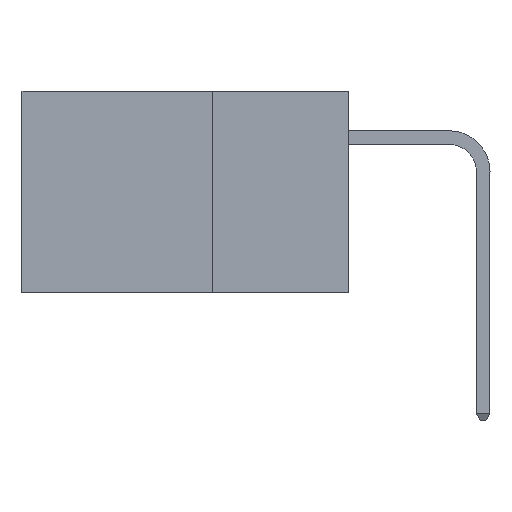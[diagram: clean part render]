
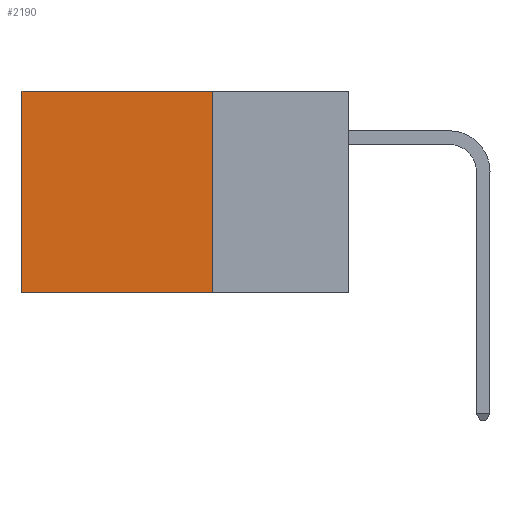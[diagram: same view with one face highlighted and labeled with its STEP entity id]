
A CAD part, left-side view. The second image highlights one B-rep face of the part: STEP entity #2190.
In plain terms, the highlighted planar face has unit normal (-1, 0, 0).
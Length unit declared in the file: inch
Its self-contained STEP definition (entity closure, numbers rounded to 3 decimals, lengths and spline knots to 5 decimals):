
#716 = CARTESIAN_POINT ( 'NONE',  ( 0.2875, 0.25, 0. ) ) ;
#831 = ORIENTED_EDGE ( 'NONE', *, *, #10721, .F. ) ;
#846 = DIRECTION ( 'NONE',  ( 0., 0., -1. ) ) ;
#870 = PLANE ( 'NONE',  #3968 ) ;
#1018 = DIRECTION ( 'NONE',  ( 1., 0., 0. ) ) ;
#1345 = ORIENTED_EDGE ( 'NONE', *, *, #7402, .T. ) ;
#1451 = EDGE_CURVE ( 'NONE', #5109, #9148, #7935, .T. ) ;
#1776 = CARTESIAN_POINT ( 'NONE',  ( 0.2875, 0.25, 0. ) ) ;
#1866 = CARTESIAN_POINT ( 'NONE',  ( 0.2875, 0.25, -0.37 ) ) ;
#1911 = DIRECTION ( 'NONE',  ( 0., 1., 0. ) ) ;
#2157 = CARTESIAN_POINT ( 'NONE',  ( 0.2875, 0.25, -0.37 ) ) ;
#2190 = ADVANCED_FACE ( 'NONE', ( #4365 ), #870, .F. ) ;
#2491 = CARTESIAN_POINT ( 'NONE',  ( 0.2875, 0.25, 0. ) ) ;
#3054 = DIRECTION ( 'NONE',  ( 0., 0., -1. ) ) ;
#3968 = AXIS2_PLACEMENT_3D ( 'NONE', #716, #1018, #846 ) ;
#4000 = DIRECTION ( 'NONE',  ( 0., 1., 0. ) ) ;
#4074 = ORIENTED_EDGE ( 'NONE', *, *, #1451, .F. ) ;
#4365 = FACE_OUTER_BOUND ( 'NONE', #11638, .T. ) ;
#4418 = VERTEX_POINT ( 'NONE', #7080 ) ;
#4975 = LINE ( 'NONE', #1776, #7325 ) ;
#5109 = VERTEX_POINT ( 'NONE', #2157 ) ;
#5740 = LINE ( 'NONE', #2491, #12959 ) ;
#6428 = CARTESIAN_POINT ( 'NONE',  ( 0.2875, 0.6, -0.37 ) ) ;
#6545 = VERTEX_POINT ( 'NONE', #7922 ) ;
#6729 = DIRECTION ( 'NONE',  ( 0., 0., -1. ) ) ;
#7080 = CARTESIAN_POINT ( 'NONE',  ( 0.2875, 0.25, 0. ) ) ;
#7325 = VECTOR ( 'NONE', #4000, 39.37008 ) ;
#7369 = EDGE_CURVE ( 'NONE', #4418, #6545, #4975, .T. ) ;
#7402 = EDGE_CURVE ( 'NONE', #6545, #9148, #9608, .T. ) ;
#7922 = CARTESIAN_POINT ( 'NONE',  ( 0.2875, 0.6, 0. ) ) ;
#7935 = LINE ( 'NONE', #1866, #10165 ) ;
#8581 = ORIENTED_EDGE ( 'NONE', *, *, #7369, .T. ) ;
#9148 = VERTEX_POINT ( 'NONE', #6428 ) ;
#9608 = LINE ( 'NONE', #11102, #12074 ) ;
#10165 = VECTOR ( 'NONE', #1911, 39.37008 ) ;
#10721 = EDGE_CURVE ( 'NONE', #4418, #5109, #5740, .T. ) ;
#11102 = CARTESIAN_POINT ( 'NONE',  ( 0.2875, 0.6, 0. ) ) ;
#11638 = EDGE_LOOP ( 'NONE', ( #1345, #4074, #831, #8581 ) ) ;
#12074 = VECTOR ( 'NONE', #3054, 39.37008 ) ;
#12959 = VECTOR ( 'NONE', #6729, 39.37008 ) ;
